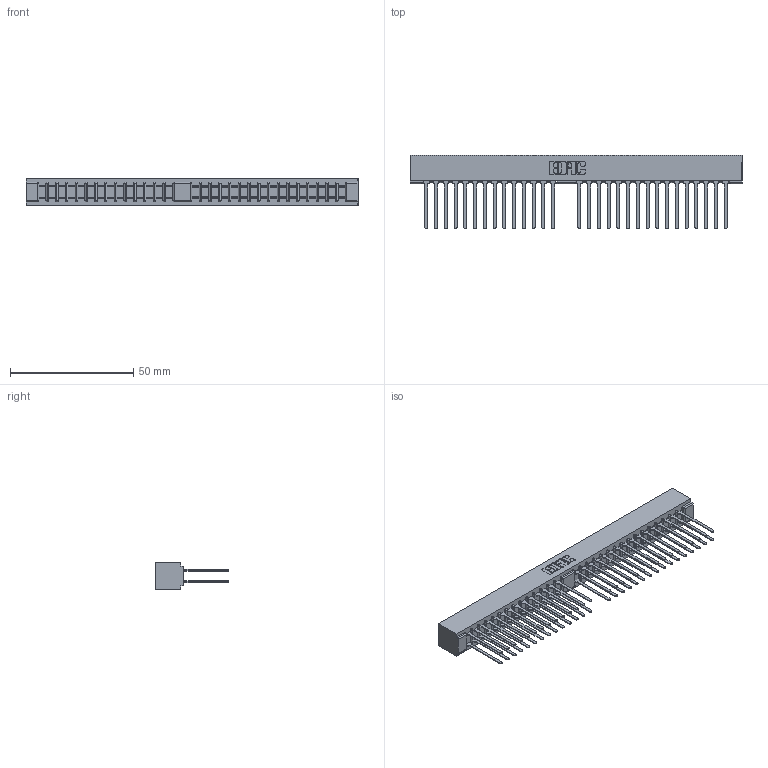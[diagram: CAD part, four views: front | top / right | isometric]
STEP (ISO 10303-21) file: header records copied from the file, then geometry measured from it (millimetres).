
FILE_DESCRIPTION (( 'STEP AP203' ), '1' );
FILE_NAME ('310-060-540-201.STEP', '2020-03-25T13:58:31', ( '' ), ( '' ), 'SwSTEP 2.0', 'SolidWorks 2016', '' );
FILE_SCHEMA (( 'CONFIG_CONTROL_DESIGN' ));
Length unit declared in the file: millimetre
Products named in the file (3): 310 Part_No Mounting Lugs; 307-290-001_540; 310-060-540-201
Assembly tree (61 placements, depth 2):
  310-060-540-201
    310 Part_No Mounting Lugs
    307-290-001_540  x60
Bounding box: 134.92 x 29.95 x 10.97 mm (x, y, z)
Volume: 12345.3 mm3; surface area: 19218.7 mm2
Topology: 61 solids, 61 shells, 2918 faces, 8137 edges, 5254 vertices
Faces by surface type: plane 1940, cylinder 914, sphere 64
Entity records: 28274 total; most frequent: CARTESIAN_POINT 4627, ORIENTED_EDGE 4582, DIRECTION 4537, EDGE_CURVE 2291, VECTOR 1761, LINE 1761, VERTEX_POINT 1478, AXIS2_PLACEMENT_3D 1388
